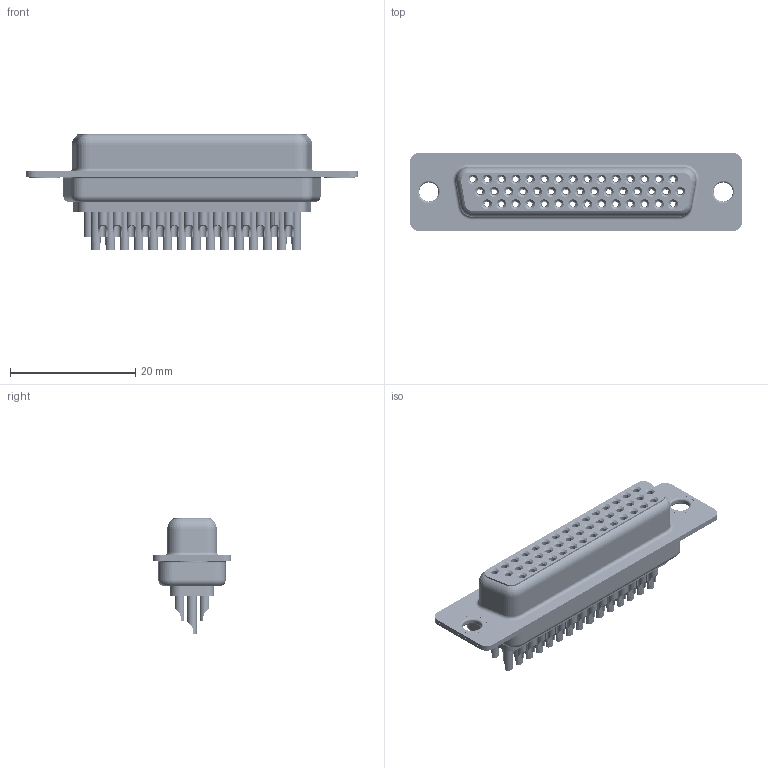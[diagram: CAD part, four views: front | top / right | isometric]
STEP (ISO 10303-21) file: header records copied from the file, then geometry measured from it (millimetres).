
FILE_DESCRIPTION (( 'STEP AP203' ), '1' );
FILE_NAME ('638-044-632-261.STEP', '2020-07-19T00:33:10', ( '' ), ( '' ), 'SwSTEP 2.0', 'SolidWorks 2020', '' );
FILE_SCHEMA (( 'CONFIG_CONTROL_DESIGN' ));
Length unit declared in the file: millimetre
Products named in the file (8): 638 Contact Row 3_32; 638 Shell Front_44 Contacts; 638 Contact Row 2_32; 638-044-632-261; 638 Thru Hole Rivet; 638 Housing_44 Contacts; 638 Shell Rear_44 Contacts; 638 Contact Row 1_32
Assembly tree (49 placements, depth 2):
  638-044-632-261
    638 Housing_44 Contacts
    638 Shell Front_44 Contacts
    638 Shell Rear_44 Contacts
    638 Contact Row 1_32  x15
    638 Contact Row 2_32  x15
    638 Contact Row 3_32  x14
    638 Thru Hole Rivet  x2
Bounding box: 53.04 x 12.6 x 18.6 mm (x, y, z)
Volume: 3265.8 mm3; surface area: 13381.3 mm2
Topology: 49 solids, 49 shells, 4169 faces, 10547 edges, 6619 vertices
Faces by surface type: cylinder 1221, plane 991, bspline 880, torus 857, cone 220
Entity records: 34244 total; most frequent: CARTESIAN_POINT 8042, DIRECTION 5436, ORIENTED_EDGE 4778, EDGE_CURVE 2389, AXIS2_PLACEMENT_3D 2298, VERTEX_POINT 1511, EDGE_LOOP 1276, CIRCLE 1273
